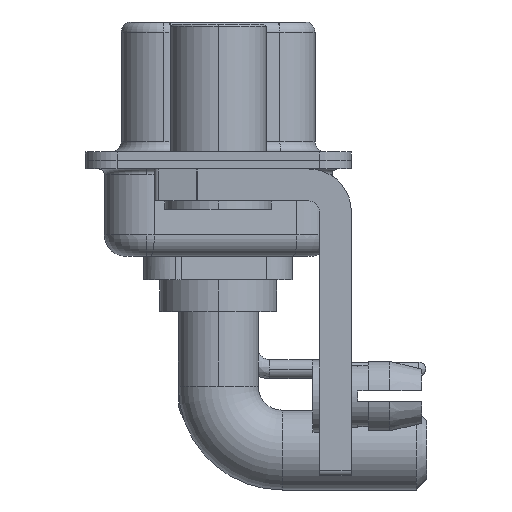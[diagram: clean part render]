
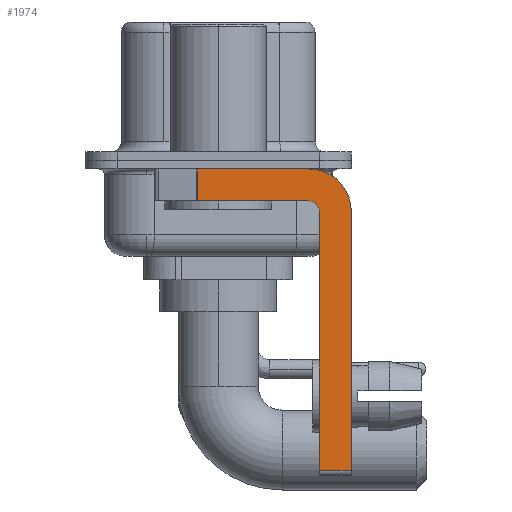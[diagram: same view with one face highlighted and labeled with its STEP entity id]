
A CAD part, left-side view. The second image highlights one B-rep face of the part: STEP entity #1974.
In plain terms, the highlighted planar face has unit normal (-1, 0, 0).
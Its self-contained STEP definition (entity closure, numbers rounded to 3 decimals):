
#1974 = ADVANCED_FACE ( 'NONE', ( #7639 ), #25171, .F. ) ;
#2023 = CARTESIAN_POINT ( 'NONE',  ( -2.9, -6.25, -2.4 ) ) ;
#2626 = LINE ( 'NONE', #5355, #3870 ) ;
#2723 = ORIENTED_EDGE ( 'NONE', *, *, #30805, .F. ) ;
#3870 = VECTOR ( 'NONE', #25033, 1000. ) ;
#4728 = CARTESIAN_POINT ( 'NONE',  ( -2.9, -4.75, -2.4 ) ) ;
#5285 = LINE ( 'NONE', #25107, #23325 ) ;
#5355 = CARTESIAN_POINT ( 'NONE',  ( -2.9, -6.25, -2.4 ) ) ;
#5926 = DIRECTION ( 'NONE',  ( 0., 0., 1. ) ) ;
#6202 = CIRCLE ( 'NONE', #10327, 0.5 ) ;
#6348 = ORIENTED_EDGE ( 'NONE', *, *, #27896, .F. ) ;
#6562 = AXIS2_PLACEMENT_3D ( 'NONE', #22588, #31838, #29572 ) ;
#6659 = VERTEX_POINT ( 'NONE', #18741 ) ;
#6983 = LINE ( 'NONE', #21606, #28827 ) ;
#7384 = CARTESIAN_POINT ( 'NONE',  ( -2.9, -6.25, -14.55 ) ) ;
#7606 = EDGE_CURVE ( 'NONE', #19841, #27275, #20284, .T. ) ;
#7639 = FACE_OUTER_BOUND ( 'NONE', #26912, .T. ) ;
#8349 = CARTESIAN_POINT ( 'NONE',  ( -2.9, 0.978, -0.4 ) ) ;
#9171 = VERTEX_POINT ( 'NONE', #7384 ) ;
#9375 = LINE ( 'NONE', #26438, #14323 ) ;
#10327 = AXIS2_PLACEMENT_3D ( 'NONE', #15822, #11113, #5926 ) ;
#10982 = ORIENTED_EDGE ( 'NONE', *, *, #31146, .T. ) ;
#11113 = DIRECTION ( 'NONE',  ( -1., 0., 0. ) ) ;
#11855 = DIRECTION ( 'NONE',  ( 0., -1., 0. ) ) ;
#12047 = LINE ( 'NONE', #12197, #13872 ) ;
#12197 = CARTESIAN_POINT ( 'NONE',  ( -2.9, 3., -0.4 ) ) ;
#12614 = ORIENTED_EDGE ( 'NONE', *, *, #14154, .T. ) ;
#12958 = ORIENTED_EDGE ( 'NONE', *, *, #19404, .F. ) ;
#13155 = ORIENTED_EDGE ( 'NONE', *, *, #31597, .F. ) ;
#13872 = VECTOR ( 'NONE', #22132, 1000. ) ;
#14154 = EDGE_CURVE ( 'NONE', #29121, #6659, #16791, .T. ) ;
#14323 = VECTOR ( 'NONE', #16681, 1000. ) ;
#15180 = DIRECTION ( 'NONE',  ( 0., 0., 1. ) ) ;
#15822 = CARTESIAN_POINT ( 'NONE',  ( -2.9, -4.25, -2.4 ) ) ;
#16651 = DIRECTION ( 'NONE',  ( 0., 0., -1. ) ) ;
#16681 = DIRECTION ( 'NONE',  ( 0., 1., 0. ) ) ;
#16791 = LINE ( 'NONE', #27030, #27932 ) ;
#17276 = DIRECTION ( 'NONE',  ( 0., 0., -1. ) ) ;
#18415 = VERTEX_POINT ( 'NONE', #4728 ) ;
#18741 = CARTESIAN_POINT ( 'NONE',  ( -2.9, 0.978, -1.9 ) ) ;
#19404 = EDGE_CURVE ( 'NONE', #22952, #18415, #5285, .T. ) ;
#19421 = CARTESIAN_POINT ( 'NONE',  ( -2.9, -4.25, -2.4 ) ) ;
#19493 = EDGE_CURVE ( 'NONE', #18415, #28077, #6202, .T. ) ;
#19606 = ORIENTED_EDGE ( 'NONE', *, *, #7606, .F. ) ;
#19841 = VERTEX_POINT ( 'NONE', #30096 ) ;
#20284 = CIRCLE ( 'NONE', #28043, 2. ) ;
#21606 = CARTESIAN_POINT ( 'NONE',  ( -2.9, -4.25, -14.55 ) ) ;
#21698 = DIRECTION ( 'NONE',  ( 1., 0., 0. ) ) ;
#22132 = DIRECTION ( 'NONE',  ( 0., -1., 0. ) ) ;
#22588 = CARTESIAN_POINT ( 'NONE',  ( -2.9, -4.25, -2.4 ) ) ;
#22952 = VERTEX_POINT ( 'NONE', #31409 ) ;
#23325 = VECTOR ( 'NONE', #15180, 1000. ) ;
#24205 = ORIENTED_EDGE ( 'NONE', *, *, #19493, .F. ) ;
#25033 = DIRECTION ( 'NONE',  ( 0., 0., -1. ) ) ;
#25107 = CARTESIAN_POINT ( 'NONE',  ( -2.9, -4.75, -14.8 ) ) ;
#25171 = PLANE ( 'NONE',  #6562 ) ;
#25336 = CARTESIAN_POINT ( 'NONE',  ( -2.9, -4.25, -1.9 ) ) ;
#26438 = CARTESIAN_POINT ( 'NONE',  ( -2.9, -4.25, -1.9 ) ) ;
#26912 = EDGE_LOOP ( 'NONE', ( #2723, #12614, #13155, #24205, #12958, #10982, #6348, #19606 ) ) ;
#27030 = CARTESIAN_POINT ( 'NONE',  ( -2.9, 0.978, -1.9 ) ) ;
#27275 = VERTEX_POINT ( 'NONE', #2023 ) ;
#27896 = EDGE_CURVE ( 'NONE', #27275, #9171, #2626, .T. ) ;
#27932 = VECTOR ( 'NONE', #17276, 1000. ) ;
#28043 = AXIS2_PLACEMENT_3D ( 'NONE', #19421, #21698, #16651 ) ;
#28077 = VERTEX_POINT ( 'NONE', #25336 ) ;
#28827 = VECTOR ( 'NONE', #11855, 1000. ) ;
#29121 = VERTEX_POINT ( 'NONE', #8349 ) ;
#29572 = DIRECTION ( 'NONE',  ( 0., 0., -1. ) ) ;
#30096 = CARTESIAN_POINT ( 'NONE',  ( -2.9, -4.25, -0.4 ) ) ;
#30805 = EDGE_CURVE ( 'NONE', #29121, #19841, #12047, .T. ) ;
#31146 = EDGE_CURVE ( 'NONE', #22952, #9171, #6983, .T. ) ;
#31409 = CARTESIAN_POINT ( 'NONE',  ( -2.9, -4.75, -14.55 ) ) ;
#31597 = EDGE_CURVE ( 'NONE', #28077, #6659, #9375, .T. ) ;
#31838 = DIRECTION ( 'NONE',  ( 1., 0., 0. ) ) ;
